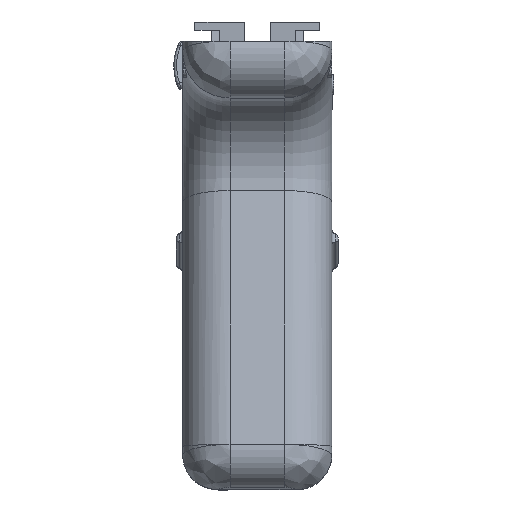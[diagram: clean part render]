
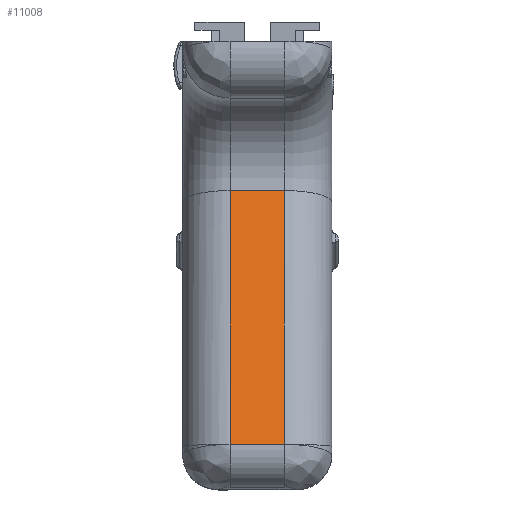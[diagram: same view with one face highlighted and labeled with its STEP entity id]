
A CAD part, front view. The second image highlights one B-rep face of the part: STEP entity #11008.
In plain terms, the highlighted face is planar.
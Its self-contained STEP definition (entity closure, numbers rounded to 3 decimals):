
#824=PLANE('',#11993);
#1320=FACE_OUTER_BOUND('',#1948,.T.);
#1948=EDGE_LOOP('',(#9501,#9502,#9503,#9504));
#2779=LINE('',#19539,#3771);
#2933=LINE('',#20306,#3925);
#2934=LINE('',#20309,#3926);
#2935=LINE('',#20310,#3927);
#3771=VECTOR('',#14127,10.);
#3925=VECTOR('',#14531,10.);
#3926=VECTOR('',#14534,10.);
#3927=VECTOR('',#14535,10.);
#5122=VERTEX_POINT('',#19535);
#5123=VERTEX_POINT('',#19537);
#5263=VERTEX_POINT('',#20282);
#5267=VERTEX_POINT('',#20308);
#6526=EDGE_CURVE('',#5122,#5123,#2779,.T.);
#6750=EDGE_CURVE('',#5122,#5263,#2933,.T.);
#6751=EDGE_CURVE('',#5267,#5123,#2934,.T.);
#6752=EDGE_CURVE('',#5263,#5267,#2935,.T.);
#9501=ORIENTED_EDGE('',*,*,#6751,.F.);
#9502=ORIENTED_EDGE('',*,*,#6752,.F.);
#9503=ORIENTED_EDGE('',*,*,#6750,.F.);
#9504=ORIENTED_EDGE('',*,*,#6526,.T.);
#11008=ADVANCED_FACE('',(#1320),#824,.T.);
#11993=AXIS2_PLACEMENT_3D('',#20307,#14532,#14533);
#14127=DIRECTION('',(0.,-0.249,0.969));
#14531=DIRECTION('',(-1.,0.,0.));
#14532=DIRECTION('center_axis',(0.,-0.969,
-0.249));
#14533=DIRECTION('ref_axis',(0.,-0.249,0.969));
#14534=DIRECTION('',(1.,0.,0.));
#14535=DIRECTION('',(0.,-0.249,0.969));
#19535=CARTESIAN_POINT('',(13.45,-69.634,19.877));
#19537=CARTESIAN_POINT('',(13.45,-81.628,66.536));
#19539=CARTESIAN_POINT('',(13.45,-81.554,66.245));
#20282=CARTESIAN_POINT('',(3.45,-69.634,19.877));
#20306=CARTESIAN_POINT('',(22.175,-69.634,19.877));
#20307=CARTESIAN_POINT('Origin',(22.175,-69.634,19.877));
#20308=CARTESIAN_POINT('',(3.45,-81.628,66.536));
#20309=CARTESIAN_POINT('',(22.175,-81.628,66.536));
#20310=CARTESIAN_POINT('',(3.45,-81.554,66.245));
